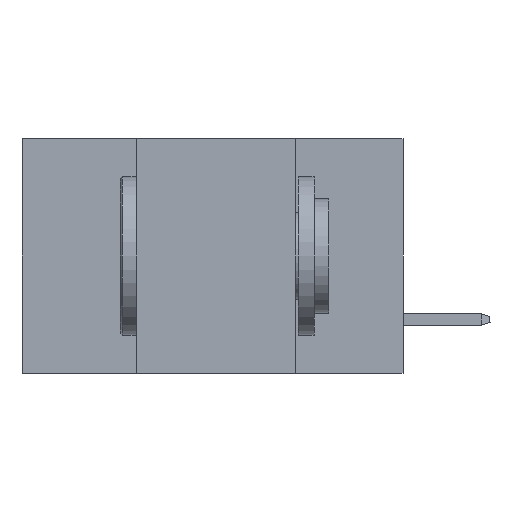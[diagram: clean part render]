
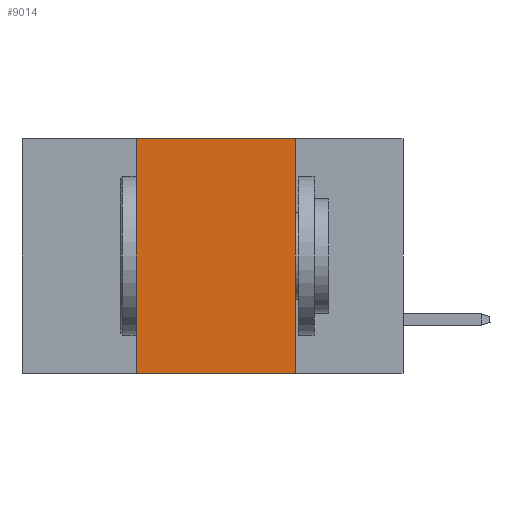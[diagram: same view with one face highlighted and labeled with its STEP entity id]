
A CAD part, left-side view. The second image highlights one B-rep face of the part: STEP entity #9014.
In plain terms, the highlighted planar face has unit normal (-1, 0, 0).
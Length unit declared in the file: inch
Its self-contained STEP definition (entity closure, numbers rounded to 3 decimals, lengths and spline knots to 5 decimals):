
#263 = VERTEX_POINT ( 'NONE', #44013 ) ;
#349 = FACE_OUTER_BOUND ( 'NONE', #22010, .T. ) ;
#2654 = VECTOR ( 'NONE', #19135, 39.37008 ) ;
#3653 = DIRECTION ( 'NONE',  ( 0., 0., -1. ) ) ;
#4347 = DIRECTION ( 'NONE',  ( 1., 0., 0. ) ) ;
#5712 = LINE ( 'NONE', #37359, #30073 ) ;
#6838 = CARTESIAN_POINT ( 'NONE',  ( 0., 0.17, 0. ) ) ;
#8116 = PLANE ( 'NONE',  #12271 ) ;
#9014 = ADVANCED_FACE ( 'NONE', ( #349 ), #8116, .F. ) ;
#9324 = VERTEX_POINT ( 'NONE', #24846 ) ;
#11746 = LINE ( 'NONE', #22124, #46028 ) ;
#12271 = AXIS2_PLACEMENT_3D ( 'NONE', #18513, #4347, #3653 ) ;
#14824 = VECTOR ( 'NONE', #25243, 39.37008 ) ;
#15057 = DIRECTION ( 'NONE',  ( 0., -1., 0. ) ) ;
#15085 = LINE ( 'NONE', #6838, #14824 ) ;
#15361 = ORIENTED_EDGE ( 'NONE', *, *, #16668, .F. ) ;
#16065 = CARTESIAN_POINT ( 'NONE',  ( 0., 0.42, 0. ) ) ;
#16305 = VERTEX_POINT ( 'NONE', #38817 ) ;
#16668 = EDGE_CURVE ( 'NONE', #16305, #263, #15085, .T. ) ;
#18363 = ORIENTED_EDGE ( 'NONE', *, *, #32664, .F. ) ;
#18513 = CARTESIAN_POINT ( 'NONE',  ( 0., 0.6, 0. ) ) ;
#19135 = DIRECTION ( 'NONE',  ( 0., 0., 1. ) ) ;
#20006 = ORIENTED_EDGE ( 'NONE', *, *, #44133, .F. ) ;
#22010 = EDGE_LOOP ( 'NONE', ( #15361, #20006, #18363, #27820 ) ) ;
#22124 = CARTESIAN_POINT ( 'NONE',  ( 0., 0.6, 0. ) ) ;
#24138 = EDGE_CURVE ( 'NONE', #9324, #263, #5712, .T. ) ;
#24846 = CARTESIAN_POINT ( 'NONE',  ( 0., 0.42, -0.37 ) ) ;
#25243 = DIRECTION ( 'NONE',  ( 0., 0., -1. ) ) ;
#27820 = ORIENTED_EDGE ( 'NONE', *, *, #24138, .T. ) ;
#30073 = VECTOR ( 'NONE', #38085, 39.37008 ) ;
#32664 = EDGE_CURVE ( 'NONE', #9324, #42945, #45137, .T. ) ;
#37359 = CARTESIAN_POINT ( 'NONE',  ( 0., 0.6, -0.37 ) ) ;
#38085 = DIRECTION ( 'NONE',  ( 0., -1., 0. ) ) ;
#38817 = CARTESIAN_POINT ( 'NONE',  ( 0., 0.17, 0. ) ) ;
#42945 = VERTEX_POINT ( 'NONE', #45050 ) ;
#44013 = CARTESIAN_POINT ( 'NONE',  ( 0., 0.17, -0.37 ) ) ;
#44133 = EDGE_CURVE ( 'NONE', #42945, #16305, #11746, .T. ) ;
#45050 = CARTESIAN_POINT ( 'NONE',  ( 0., 0.42, 0. ) ) ;
#45137 = LINE ( 'NONE', #16065, #2654 ) ;
#46028 = VECTOR ( 'NONE', #15057, 39.37008 ) ;
